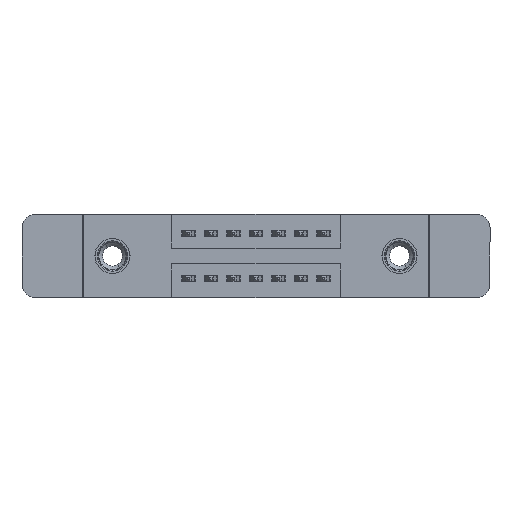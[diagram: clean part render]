
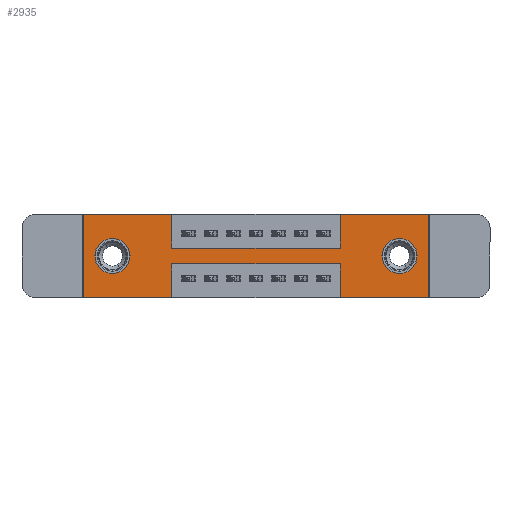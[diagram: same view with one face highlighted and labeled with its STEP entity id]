
A CAD part, front view. The second image highlights one B-rep face of the part: STEP entity #2935.
In plain terms, the highlighted planar face has unit normal (0, -1, 0).
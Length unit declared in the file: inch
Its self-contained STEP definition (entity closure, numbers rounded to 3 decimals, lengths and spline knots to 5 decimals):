
#4 = CARTESIAN_POINT ( 'NONE',  ( 0.13, 0., -0.185 ) ) ;
#120 = ORIENTED_EDGE ( 'NONE', *, *, #14918, .T. ) ;
#136 = ORIENTED_EDGE ( 'NONE', *, *, #202, .F. ) ;
#144 = DIRECTION ( 'NONE',  ( -1., 0., 0. ) ) ;
#155 = VECTOR ( 'NONE', #15384, 39.37008 ) ;
#179 = AXIS2_PLACEMENT_3D ( 'NONE', #14629, #7649, #353 ) ;
#202 = EDGE_CURVE ( 'NONE', #838, #11043, #10573, .T. ) ;
#353 = DIRECTION ( 'NONE',  ( 0., 0., 1. ) ) ;
#444 = EDGE_CURVE ( 'NONE', #11324, #838, #1745, .T. ) ;
#604 = VERTEX_POINT ( 'NONE', #6510 ) ;
#633 = FACE_BOUND ( 'NONE', #4252, .T. ) ;
#665 = CIRCLE ( 'NONE', #11973, 0.078 ) ;
#725 = CIRCLE ( 'NONE', #7509, 0.078 ) ;
#760 = VERTEX_POINT ( 'NONE', #4237 ) ;
#838 = VERTEX_POINT ( 'NONE', #3667 ) ;
#994 = AXIS2_PLACEMENT_3D ( 'NONE', #1733, #1730, #1714 ) ;
#1065 = VECTOR ( 'NONE', #9014, 39.37008 ) ;
#1081 = EDGE_CURVE ( 'NONE', #8433, #760, #12918, .T. ) ;
#1203 = CARTESIAN_POINT ( 'NONE',  ( 1.1425, 0., -0.37 ) ) ;
#1218 = EDGE_CURVE ( 'NONE', #2503, #6514, #725, .T. ) ;
#1300 = DIRECTION ( 'NONE',  ( 0., 0., 1. ) ) ;
#1419 = CARTESIAN_POINT ( 'NONE',  ( 1.535, 0., -0.37 ) ) ;
#1572 = VECTOR ( 'NONE', #9238, 39.37008 ) ;
#1714 = DIRECTION ( 'NONE',  ( 0., 0., -1. ) ) ;
#1730 = DIRECTION ( 'NONE',  ( 0., 1., 0. ) ) ;
#1733 = CARTESIAN_POINT ( 'NONE',  ( 1.405, 0., -0.185 ) ) ;
#1745 = LINE ( 'NONE', #7885, #13302 ) ;
#1950 = LINE ( 'NONE', #3387, #5185 ) ;
#1969 = EDGE_CURVE ( 'NONE', #8794, #11324, #5325, .T. ) ;
#1999 = CARTESIAN_POINT ( 'NONE',  ( 0., 0., 0. ) ) ;
#2028 = CARTESIAN_POINT ( 'NONE',  ( 1.535, 0., 0. ) ) ;
#2161 = EDGE_LOOP ( 'NONE', ( #13249, #11307 ) ) ;
#2269 = CARTESIAN_POINT ( 'NONE',  ( 0.3925, 0., -0.37 ) ) ;
#2463 = ORIENTED_EDGE ( 'NONE', *, *, #1969, .F. ) ;
#2503 = VERTEX_POINT ( 'NONE', #15431 ) ;
#2876 = LINE ( 'NONE', #10101, #5701 ) ;
#2935 = ADVANCED_FACE ( 'NONE', ( #633, #4670, #13005 ), #12777, .T. ) ;
#3015 = CARTESIAN_POINT ( 'NONE',  ( 1.535, 0., 0. ) ) ;
#3387 = CARTESIAN_POINT ( 'NONE',  ( 0., 0., -0.37 ) ) ;
#3667 = CARTESIAN_POINT ( 'NONE',  ( 0., 0., -0.37 ) ) ;
#3820 = VERTEX_POINT ( 'NONE', #1419 ) ;
#4005 = CARTESIAN_POINT ( 'NONE',  ( 0., 0., 0. ) ) ;
#4141 = LINE ( 'NONE', #15127, #6938 ) ;
#4237 = CARTESIAN_POINT ( 'NONE',  ( 1.405, 0., -0.263 ) ) ;
#4252 = EDGE_LOOP ( 'NONE', ( #6237, #120 ) ) ;
#4261 = CARTESIAN_POINT ( 'NONE',  ( 1.1425, 0., 0. ) ) ;
#4282 = CARTESIAN_POINT ( 'NONE',  ( 1.405, 0., -0.185 ) ) ;
#4326 = CARTESIAN_POINT ( 'NONE',  ( 1.1425, 0., -0.15 ) ) ;
#4439 = CARTESIAN_POINT ( 'NONE',  ( 1.405, 0., -0.107 ) ) ;
#4670 = FACE_BOUND ( 'NONE', #2161, .T. ) ;
#4682 = DIRECTION ( 'NONE',  ( 0., 0., 1. ) ) ;
#5007 = EDGE_CURVE ( 'NONE', #8063, #14958, #12795, .T. ) ;
#5042 = CARTESIAN_POINT ( 'NONE',  ( 0.3925, 0., -0.37 ) ) ;
#5090 = CARTESIAN_POINT ( 'NONE',  ( 0.3925, 0., -0.22 ) ) ;
#5185 = VECTOR ( 'NONE', #6969, 39.37008 ) ;
#5325 = LINE ( 'NONE', #5042, #14324 ) ;
#5501 = DIRECTION ( 'NONE',  ( 0., 0., -1. ) ) ;
#5701 = VECTOR ( 'NONE', #11315, 39.37008 ) ;
#5863 = EDGE_CURVE ( 'NONE', #10642, #10770, #13863, .T. ) ;
#6053 = ORIENTED_EDGE ( 'NONE', *, *, #14723, .F. ) ;
#6237 = ORIENTED_EDGE ( 'NONE', *, *, #1081, .T. ) ;
#6250 = DIRECTION ( 'NONE',  ( 0., 0., -1. ) ) ;
#6279 = LINE ( 'NONE', #13093, #155 ) ;
#6424 = DIRECTION ( 'NONE',  ( 1., 0., 0. ) ) ;
#6510 = CARTESIAN_POINT ( 'NONE',  ( 0.3925, 0., 0. ) ) ;
#6514 = VERTEX_POINT ( 'NONE', #6940 ) ;
#6740 = DIRECTION ( 'NONE',  ( 0., 1., 0. ) ) ;
#6938 = VECTOR ( 'NONE', #8141, 39.37008 ) ;
#6940 = CARTESIAN_POINT ( 'NONE',  ( 0.13, 0., -0.263 ) ) ;
#6941 = DIRECTION ( 'NONE',  ( 0., 0., -1. ) ) ;
#6969 = DIRECTION ( 'NONE',  ( -1., 0., 0. ) ) ;
#7509 = AXIS2_PLACEMENT_3D ( 'NONE', #4, #6740, #1300 ) ;
#7564 = ORIENTED_EDGE ( 'NONE', *, *, #8895, .F. ) ;
#7649 = DIRECTION ( 'NONE',  ( 0., 1., 0. ) ) ;
#7872 = DIRECTION ( 'NONE',  ( -1., 0., 0. ) ) ;
#7885 = CARTESIAN_POINT ( 'NONE',  ( 0., 0., -0.37 ) ) ;
#7959 = ORIENTED_EDGE ( 'NONE', *, *, #5863, .F. ) ;
#8063 = VERTEX_POINT ( 'NONE', #14353 ) ;
#8112 = LINE ( 'NONE', #12967, #13218 ) ;
#8141 = DIRECTION ( 'NONE',  ( 1., 0., 0. ) ) ;
#8336 = ORIENTED_EDGE ( 'NONE', *, *, #9141, .F. ) ;
#8433 = VERTEX_POINT ( 'NONE', #4439 ) ;
#8668 = VECTOR ( 'NONE', #144, 39.37008 ) ;
#8719 = VERTEX_POINT ( 'NONE', #14484 ) ;
#8794 = VERTEX_POINT ( 'NONE', #9991 ) ;
#8802 = EDGE_CURVE ( 'NONE', #6514, #2503, #14124, .T. ) ;
#8895 = EDGE_CURVE ( 'NONE', #10770, #3820, #13041, .T. ) ;
#9014 = DIRECTION ( 'NONE',  ( 0., 0., -1. ) ) ;
#9141 = EDGE_CURVE ( 'NONE', #14958, #10642, #8112, .T. ) ;
#9238 = DIRECTION ( 'NONE',  ( 1., 0., 0. ) ) ;
#9990 = ORIENTED_EDGE ( 'NONE', *, *, #13109, .F. ) ;
#9991 = CARTESIAN_POINT ( 'NONE',  ( 0.3925, 0., -0.22 ) ) ;
#10033 = AXIS2_PLACEMENT_3D ( 'NONE', #11691, #13986, #6941 ) ;
#10101 = CARTESIAN_POINT ( 'NONE',  ( 1.1425, 0., -0.37 ) ) ;
#10573 = LINE ( 'NONE', #11106, #13645 ) ;
#10642 = VERTEX_POINT ( 'NONE', #4261 ) ;
#10770 = VERTEX_POINT ( 'NONE', #2028 ) ;
#11043 = VERTEX_POINT ( 'NONE', #4005 ) ;
#11106 = CARTESIAN_POINT ( 'NONE',  ( 0., 0., 0. ) ) ;
#11184 = DIRECTION ( 'NONE',  ( 0., 0., 1. ) ) ;
#11307 = ORIENTED_EDGE ( 'NONE', *, *, #8802, .T. ) ;
#11311 = EDGE_CURVE ( 'NONE', #3820, #14012, #1950, .T. ) ;
#11315 = DIRECTION ( 'NONE',  ( 0., 0., 1. ) ) ;
#11324 = VERTEX_POINT ( 'NONE', #2269 ) ;
#11484 = ORIENTED_EDGE ( 'NONE', *, *, #5007, .F. ) ;
#11691 = CARTESIAN_POINT ( 'NONE',  ( 0., 0., -0.37 ) ) ;
#11973 = AXIS2_PLACEMENT_3D ( 'NONE', #4282, #12594, #5501 ) ;
#12460 = VECTOR ( 'NONE', #6424, 39.37008 ) ;
#12556 = ORIENTED_EDGE ( 'NONE', *, *, #15094, .F. ) ;
#12594 = DIRECTION ( 'NONE',  ( 0., 1., 0. ) ) ;
#12777 = PLANE ( 'NONE',  #10033 ) ;
#12795 = LINE ( 'NONE', #14610, #12460 ) ;
#12868 = EDGE_CURVE ( 'NONE', #604, #8063, #6279, .T. ) ;
#12918 = CIRCLE ( 'NONE', #994, 0.078 ) ;
#12963 = EDGE_LOOP ( 'NONE', ( #2463, #6053, #9990, #13070, #7564, #7959, #8336, #11484, #14856, #12556, #136, #13262 ) ) ;
#12967 = CARTESIAN_POINT ( 'NONE',  ( 1.1425, 0., 0. ) ) ;
#13005 = FACE_OUTER_BOUND ( 'NONE', #12963, .T. ) ;
#13041 = LINE ( 'NONE', #3015, #1065 ) ;
#13070 = ORIENTED_EDGE ( 'NONE', *, *, #11311, .F. ) ;
#13093 = CARTESIAN_POINT ( 'NONE',  ( 0.3925, 0., 0. ) ) ;
#13109 = EDGE_CURVE ( 'NONE', #14012, #8719, #2876, .T. ) ;
#13218 = VECTOR ( 'NONE', #4682, 39.37008 ) ;
#13249 = ORIENTED_EDGE ( 'NONE', *, *, #1218, .T. ) ;
#13262 = ORIENTED_EDGE ( 'NONE', *, *, #444, .F. ) ;
#13302 = VECTOR ( 'NONE', #7872, 39.37008 ) ;
#13645 = VECTOR ( 'NONE', #11184, 39.37008 ) ;
#13863 = LINE ( 'NONE', #1999, #1572 ) ;
#13986 = DIRECTION ( 'NONE',  ( 0., -1., 0. ) ) ;
#14012 = VERTEX_POINT ( 'NONE', #1203 ) ;
#14124 = CIRCLE ( 'NONE', #179, 0.078 ) ;
#14324 = VECTOR ( 'NONE', #6250, 39.37008 ) ;
#14353 = CARTESIAN_POINT ( 'NONE',  ( 0.3925, 0., -0.15 ) ) ;
#14484 = CARTESIAN_POINT ( 'NONE',  ( 1.1425, 0., -0.22 ) ) ;
#14610 = CARTESIAN_POINT ( 'NONE',  ( 0.3925, 0., -0.15 ) ) ;
#14629 = CARTESIAN_POINT ( 'NONE',  ( 0.13, 0., -0.185 ) ) ;
#14723 = EDGE_CURVE ( 'NONE', #8719, #8794, #15179, .T. ) ;
#14856 = ORIENTED_EDGE ( 'NONE', *, *, #12868, .F. ) ;
#14918 = EDGE_CURVE ( 'NONE', #760, #8433, #665, .T. ) ;
#14958 = VERTEX_POINT ( 'NONE', #4326 ) ;
#15094 = EDGE_CURVE ( 'NONE', #11043, #604, #4141, .T. ) ;
#15127 = CARTESIAN_POINT ( 'NONE',  ( 0., 0., 0. ) ) ;
#15179 = LINE ( 'NONE', #5090, #8668 ) ;
#15384 = DIRECTION ( 'NONE',  ( 0., 0., -1. ) ) ;
#15431 = CARTESIAN_POINT ( 'NONE',  ( 0.13, 0., -0.107 ) ) ;
